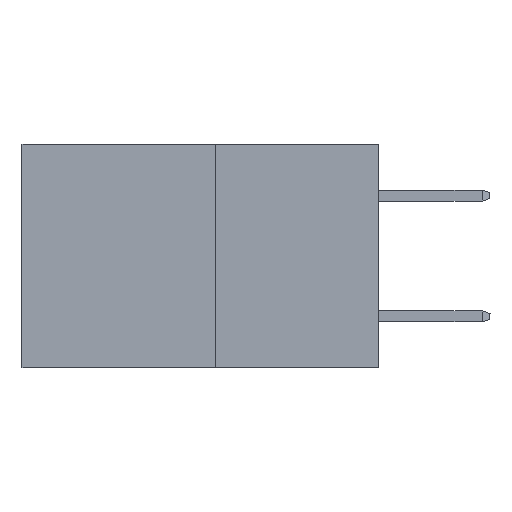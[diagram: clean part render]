
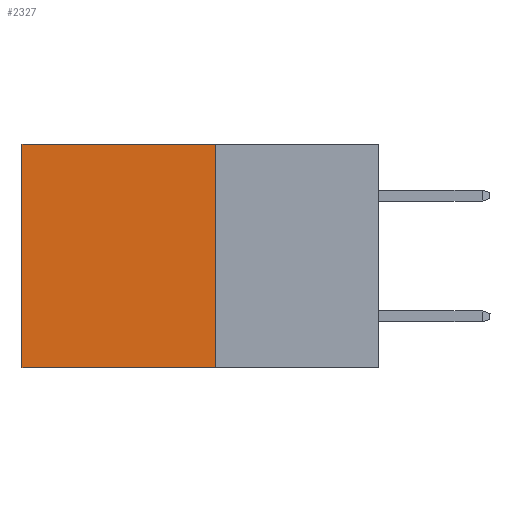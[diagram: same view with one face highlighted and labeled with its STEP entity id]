
A CAD part, left-side view. The second image highlights one B-rep face of the part: STEP entity #2327.
In plain terms, the highlighted planar face has unit normal (-1, 0, 0).
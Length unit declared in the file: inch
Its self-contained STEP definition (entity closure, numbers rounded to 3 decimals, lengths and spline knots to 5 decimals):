
#146 = CARTESIAN_POINT ( 'NONE',  ( 0.277, 0.27, -0.37 ) ) ;
#244 = DIRECTION ( 'NONE',  ( 0., 0., -1. ) ) ;
#255 = DIRECTION ( 'NONE',  ( 1., 0., 0. ) ) ;
#442 = EDGE_CURVE ( 'NONE', #8966, #1833, #5524, .T. ) ;
#466 = VECTOR ( 'NONE', #9707, 39.37008 ) ;
#648 = VERTEX_POINT ( 'NONE', #3248 ) ;
#1226 = VECTOR ( 'NONE', #9337, 39.37008 ) ;
#1833 = VERTEX_POINT ( 'NONE', #2653 ) ;
#1945 = CARTESIAN_POINT ( 'NONE',  ( 0.277, 0.27, -0.37 ) ) ;
#2327 = ADVANCED_FACE ( 'NONE', ( #8800 ), #3303, .F. ) ;
#2518 = LINE ( 'NONE', #9814, #466 ) ;
#2653 = CARTESIAN_POINT ( 'NONE',  ( 0.277, 0.59, 0. ) ) ;
#3061 = ORIENTED_EDGE ( 'NONE', *, *, #6540, .F. ) ;
#3181 = LINE ( 'NONE', #7622, #6916 ) ;
#3248 = CARTESIAN_POINT ( 'NONE',  ( 0.277, 0.59, -0.37 ) ) ;
#3303 = PLANE ( 'NONE',  #9379 ) ;
#3507 = EDGE_CURVE ( 'NONE', #8304, #648, #6857, .T. ) ;
#5346 = ORIENTED_EDGE ( 'NONE', *, *, #6137, .T. ) ;
#5524 = LINE ( 'NONE', #9114, #1226 ) ;
#6137 = EDGE_CURVE ( 'NONE', #1833, #648, #3181, .T. ) ;
#6540 = EDGE_CURVE ( 'NONE', #8966, #8304, #2518, .T. ) ;
#6546 = DIRECTION ( 'NONE',  ( 0., 1., 0. ) ) ;
#6617 = DIRECTION ( 'NONE',  ( 0., 0., -1. ) ) ;
#6857 = LINE ( 'NONE', #7505, #8123 ) ;
#6916 = VECTOR ( 'NONE', #6617, 39.37008 ) ;
#7505 = CARTESIAN_POINT ( 'NONE',  ( 0.277, 0.27, -0.37 ) ) ;
#7622 = CARTESIAN_POINT ( 'NONE',  ( 0.277, 0.59, -0.37 ) ) ;
#7952 = ORIENTED_EDGE ( 'NONE', *, *, #442, .T. ) ;
#8123 = VECTOR ( 'NONE', #6546, 39.37008 ) ;
#8304 = VERTEX_POINT ( 'NONE', #1945 ) ;
#8705 = ORIENTED_EDGE ( 'NONE', *, *, #3507, .F. ) ;
#8800 = FACE_OUTER_BOUND ( 'NONE', #9307, .T. ) ;
#8966 = VERTEX_POINT ( 'NONE', #9744 ) ;
#9114 = CARTESIAN_POINT ( 'NONE',  ( 0.277, 0.27, 0. ) ) ;
#9307 = EDGE_LOOP ( 'NONE', ( #5346, #8705, #3061, #7952 ) ) ;
#9337 = DIRECTION ( 'NONE',  ( 0., 1., 0. ) ) ;
#9379 = AXIS2_PLACEMENT_3D ( 'NONE', #146, #255, #244 ) ;
#9707 = DIRECTION ( 'NONE',  ( 0., 0., -1. ) ) ;
#9744 = CARTESIAN_POINT ( 'NONE',  ( 0.277, 0.27, 0. ) ) ;
#9814 = CARTESIAN_POINT ( 'NONE',  ( 0.277, 0.27, -0.37 ) ) ;
